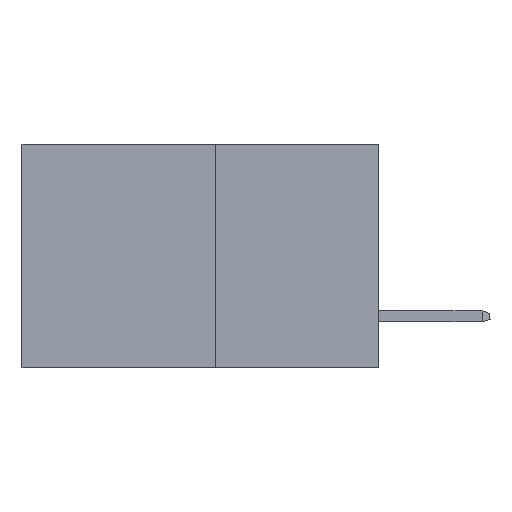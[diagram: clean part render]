
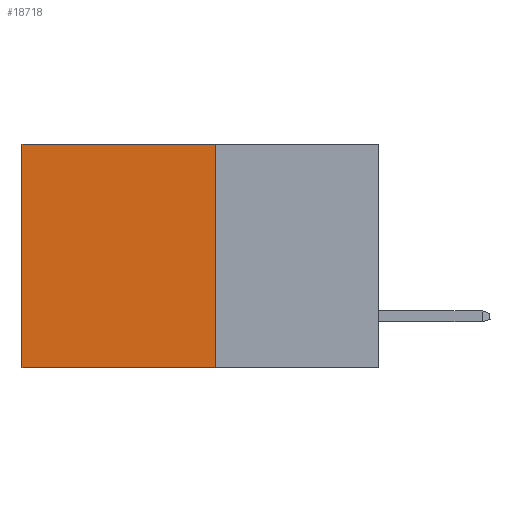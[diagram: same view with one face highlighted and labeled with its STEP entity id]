
A CAD part, left-side view. The second image highlights one B-rep face of the part: STEP entity #18718.
In plain terms, the highlighted planar face has unit normal (-1, 0, 0).
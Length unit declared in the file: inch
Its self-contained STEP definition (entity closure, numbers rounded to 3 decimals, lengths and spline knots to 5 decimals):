
#37 = LINE ( 'NONE', #9112, #8914 ) ;
#973 = DIRECTION ( 'NONE',  ( 0., 1., 0. ) ) ;
#1107 = VECTOR ( 'NONE', #7501, 39.37008 ) ;
#1158 = CARTESIAN_POINT ( 'NONE',  ( 0.277, 0.59, -0.37 ) ) ;
#1590 = CARTESIAN_POINT ( 'NONE',  ( 0.277, 0.59, 0. ) ) ;
#2071 = CARTESIAN_POINT ( 'NONE',  ( 0.277, 0.27, -0.37 ) ) ;
#2108 = VECTOR ( 'NONE', #15153, 39.37008 ) ;
#2194 = DIRECTION ( 'NONE',  ( 0., 1., 0. ) ) ;
#2447 = CARTESIAN_POINT ( 'NONE',  ( 0.277, 0.27, -0.37 ) ) ;
#3232 = LINE ( 'NONE', #1158, #2108 ) ;
#4243 = DIRECTION ( 'NONE',  ( 0., 0., -1. ) ) ;
#4330 = EDGE_LOOP ( 'NONE', ( #14412, #17143, #11022, #8797 ) ) ;
#4812 = EDGE_CURVE ( 'NONE', #5285, #15058, #37, .T. ) ;
#5285 = VERTEX_POINT ( 'NONE', #6973 ) ;
#5384 = VECTOR ( 'NONE', #973, 39.37008 ) ;
#6973 = CARTESIAN_POINT ( 'NONE',  ( 0.277, 0.27, 0. ) ) ;
#7501 = DIRECTION ( 'NONE',  ( 0., 0., -1. ) ) ;
#7688 = PLANE ( 'NONE',  #8687 ) ;
#8687 = AXIS2_PLACEMENT_3D ( 'NONE', #2447, #14661, #4243 ) ;
#8797 = ORIENTED_EDGE ( 'NONE', *, *, #4812, .T. ) ;
#8914 = VECTOR ( 'NONE', #2194, 39.37008 ) ;
#9112 = CARTESIAN_POINT ( 'NONE',  ( 0.277, 0.27, 0. ) ) ;
#9758 = CARTESIAN_POINT ( 'NONE',  ( 0.277, 0.27, -0.37 ) ) ;
#10005 = LINE ( 'NONE', #9758, #5384 ) ;
#11022 = ORIENTED_EDGE ( 'NONE', *, *, #21048, .F. ) ;
#11229 = EDGE_CURVE ( 'NONE', #15058, #11815, #3232, .T. ) ;
#11815 = VERTEX_POINT ( 'NONE', #18185 ) ;
#12348 = EDGE_CURVE ( 'NONE', #21701, #11815, #10005, .T. ) ;
#14388 = CARTESIAN_POINT ( 'NONE',  ( 0.277, 0.27, -0.37 ) ) ;
#14412 = ORIENTED_EDGE ( 'NONE', *, *, #11229, .T. ) ;
#14661 = DIRECTION ( 'NONE',  ( 1., 0., 0. ) ) ;
#15058 = VERTEX_POINT ( 'NONE', #1590 ) ;
#15153 = DIRECTION ( 'NONE',  ( 0., 0., -1. ) ) ;
#15956 = FACE_OUTER_BOUND ( 'NONE', #4330, .T. ) ;
#17143 = ORIENTED_EDGE ( 'NONE', *, *, #12348, .F. ) ;
#18185 = CARTESIAN_POINT ( 'NONE',  ( 0.277, 0.59, -0.37 ) ) ;
#18718 = ADVANCED_FACE ( 'NONE', ( #15956 ), #7688, .F. ) ;
#19601 = LINE ( 'NONE', #14388, #1107 ) ;
#21048 = EDGE_CURVE ( 'NONE', #5285, #21701, #19601, .T. ) ;
#21701 = VERTEX_POINT ( 'NONE', #2071 ) ;
